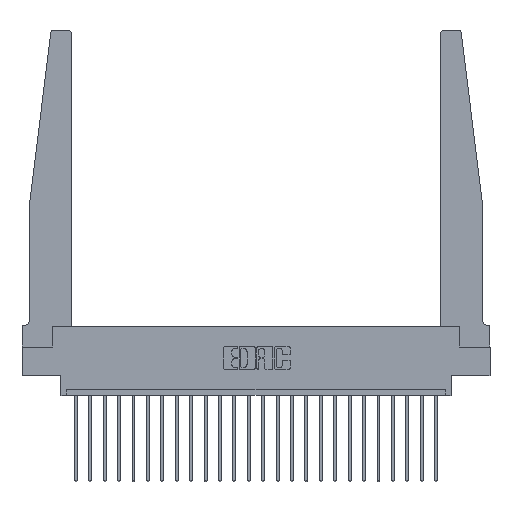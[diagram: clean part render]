
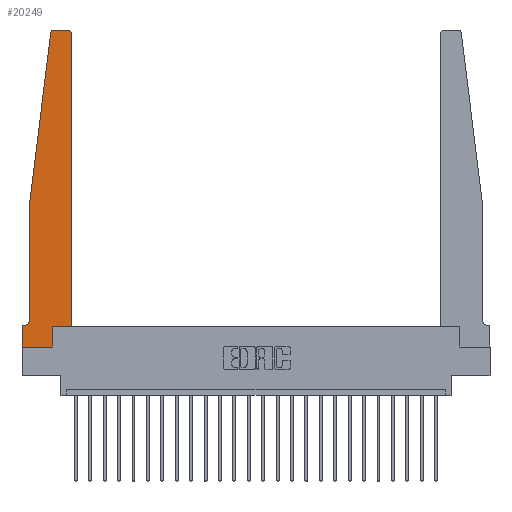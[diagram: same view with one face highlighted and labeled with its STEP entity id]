
A CAD part, top view. The second image highlights one B-rep face of the part: STEP entity #20249.
In plain terms, the highlighted planar face has unit normal (0, 0, 1).
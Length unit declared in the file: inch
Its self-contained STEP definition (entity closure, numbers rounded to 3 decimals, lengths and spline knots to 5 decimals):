
#148 = CARTESIAN_POINT ( 'NONE',  ( 0.24675, 2.72367, 0.37 ) ) ;
#236 = LINE ( 'NONE', #5262, #6137 ) ;
#326 = VERTEX_POINT ( 'NONE', #9006 ) ;
#773 = LINE ( 'NONE', #8058, #2412 ) ;
#903 = VERTEX_POINT ( 'NONE', #23193 ) ;
#1017 = ORIENTED_EDGE ( 'NONE', *, *, #5343, .T. ) ;
#1084 = VERTEX_POINT ( 'NONE', #5472 ) ;
#1524 = EDGE_CURVE ( 'NONE', #8027, #1084, #5301, .T. ) ;
#1527 = EDGE_CURVE ( 'NONE', #903, #20005, #21929, .T. ) ;
#1759 = VERTEX_POINT ( 'NONE', #4455 ) ;
#1843 = CARTESIAN_POINT ( 'NONE',  ( 0.2605, 0., 0.37 ) ) ;
#1944 = CARTESIAN_POINT ( 'NONE',  ( 0., 0., 0.37 ) ) ;
#2383 = DIRECTION ( 'NONE',  ( 0., 1., 0. ) ) ;
#2412 = VECTOR ( 'NONE', #18839, 39.37008 ) ;
#2523 = VECTOR ( 'NONE', #2383, 39.37008 ) ;
#2601 = CARTESIAN_POINT ( 'NONE',  ( 0.065, 0.1875, 0.37 ) ) ;
#2729 = DIRECTION ( 'NONE',  ( 0., 0., 1. ) ) ;
#2732 = DIRECTION ( 'NONE',  ( 0., 0., 1. ) ) ;
#2980 = CARTESIAN_POINT ( 'NONE',  ( 0.27653, 2.72, 0.37 ) ) ;
#3102 = EDGE_CURVE ( 'NONE', #5681, #13576, #7999, .T. ) ;
#3300 = CARTESIAN_POINT ( 'NONE',  ( 0., 0.1875, 0.37 ) ) ;
#3332 = VECTOR ( 'NONE', #19540, 39.37008 ) ;
#3386 = ORIENTED_EDGE ( 'NONE', *, *, #1524, .T. ) ;
#3701 = VECTOR ( 'NONE', #3868, 39.37008 ) ;
#3868 = DIRECTION ( 'NONE',  ( 0., -1., 0. ) ) ;
#3895 = EDGE_CURVE ( 'NONE', #1759, #903, #12063, .T. ) ;
#4279 = EDGE_CURVE ( 'NONE', #1084, #1759, #20562, .T. ) ;
#4455 = CARTESIAN_POINT ( 'NONE',  ( 0.015, 0.1875, 0.37 ) ) ;
#4622 = VERTEX_POINT ( 'NONE', #4796 ) ;
#4790 = CIRCLE ( 'NONE', #18169, 0.03 ) ;
#4796 = CARTESIAN_POINT ( 'NONE',  ( 0.395, 2.75, 0.37 ) ) ;
#4825 = DIRECTION ( 'NONE',  ( -1., 0., 0. ) ) ;
#4871 = FACE_OUTER_BOUND ( 'NONE', #10097, .T. ) ;
#5262 = CARTESIAN_POINT ( 'NONE',  ( 0.425, 0.18, 0.37 ) ) ;
#5301 = LINE ( 'NONE', #5767, #3701 ) ;
#5343 = EDGE_CURVE ( 'NONE', #20005, #5681, #11572, .T. ) ;
#5472 = CARTESIAN_POINT ( 'NONE',  ( 0.065, 0.2375, 0.37 ) ) ;
#5681 = VERTEX_POINT ( 'NONE', #1843 ) ;
#5767 = CARTESIAN_POINT ( 'NONE',  ( 0.065, 1.25, 0.37 ) ) ;
#6028 = LINE ( 'NONE', #11548, #22007 ) ;
#6137 = VECTOR ( 'NONE', #16498, 39.37008 ) ;
#6341 = VECTOR ( 'NONE', #23479, 39.37008 ) ;
#6437 = EDGE_CURVE ( 'NONE', #326, #4622, #4790, .T. ) ;
#7247 = EDGE_CURVE ( 'NONE', #19498, #8027, #6028, .T. ) ;
#7261 = AXIS2_PLACEMENT_3D ( 'NONE', #2980, #2732, #10279 ) ;
#7490 = ORIENTED_EDGE ( 'NONE', *, *, #1527, .T. ) ;
#7635 = CIRCLE ( 'NONE', #7261, 0.03 ) ;
#7999 = LINE ( 'NONE', #11383, #2523 ) ;
#8027 = VERTEX_POINT ( 'NONE', #22631 ) ;
#8058 = CARTESIAN_POINT ( 'NONE',  ( 0.25, 2.75, 0.37 ) ) ;
#8217 = DIRECTION ( 'NONE',  ( -1., 0., 0. ) ) ;
#9006 = CARTESIAN_POINT ( 'NONE',  ( 0.425, 2.72, 0.37 ) ) ;
#9083 = ORIENTED_EDGE ( 'NONE', *, *, #3102, .T. ) ;
#9211 = ORIENTED_EDGE ( 'NONE', *, *, #21481, .T. ) ;
#9898 = CARTESIAN_POINT ( 'NONE',  ( 0.425, 0.18, 0.37 ) ) ;
#10097 = EDGE_LOOP ( 'NONE', ( #18617, #9211, #16314, #3386, #12042, #16622, #7490, #1017, #9083, #17305, #13920, #22218 ) ) ;
#10279 = DIRECTION ( 'NONE',  ( 1., 0., 0. ) ) ;
#11383 = CARTESIAN_POINT ( 'NONE',  ( 0.2605, 0.18, 0.37 ) ) ;
#11409 = EDGE_CURVE ( 'NONE', #4622, #19148, #773, .T. ) ;
#11443 = AXIS2_PLACEMENT_3D ( 'NONE', #3300, #17546, #21727 ) ;
#11548 = CARTESIAN_POINT ( 'NONE',  ( 0.065, 1.25, 0.37 ) ) ;
#11572 = LINE ( 'NONE', #22678, #14547 ) ;
#12042 = ORIENTED_EDGE ( 'NONE', *, *, #4279, .T. ) ;
#12063 = LINE ( 'NONE', #2601, #19394 ) ;
#12240 = DIRECTION ( 'NONE',  ( 0., 0., -1. ) ) ;
#12656 = DIRECTION ( 'NONE',  ( 1., 0., 0. ) ) ;
#13576 = VERTEX_POINT ( 'NONE', #20661 ) ;
#13697 = DIRECTION ( 'NONE',  ( -0.122, -0.992, 0. ) ) ;
#13920 = ORIENTED_EDGE ( 'NONE', *, *, #23523, .T. ) ;
#14271 = CARTESIAN_POINT ( 'NONE',  ( 0.425, 0.18, 0.37 ) ) ;
#14547 = VECTOR ( 'NONE', #19206, 39.37008 ) ;
#15595 = VERTEX_POINT ( 'NONE', #9898 ) ;
#16314 = ORIENTED_EDGE ( 'NONE', *, *, #7247, .T. ) ;
#16498 = DIRECTION ( 'NONE',  ( 0., 1., 0. ) ) ;
#16622 = ORIENTED_EDGE ( 'NONE', *, *, #3895, .T. ) ;
#17305 = ORIENTED_EDGE ( 'NONE', *, *, #17995, .T. ) ;
#17431 = CARTESIAN_POINT ( 'NONE',  ( 0., 0., 0.37 ) ) ;
#17546 = DIRECTION ( 'NONE',  ( 0., 0., 1. ) ) ;
#17861 = LINE ( 'NONE', #14271, #3332 ) ;
#17995 = EDGE_CURVE ( 'NONE', #13576, #15595, #17861, .T. ) ;
#18021 = PLANE ( 'NONE',  #11443 ) ;
#18169 = AXIS2_PLACEMENT_3D ( 'NONE', #19118, #2729, #12656 ) ;
#18617 = ORIENTED_EDGE ( 'NONE', *, *, #11409, .T. ) ;
#18839 = DIRECTION ( 'NONE',  ( -1., 0., 0. ) ) ;
#19118 = CARTESIAN_POINT ( 'NONE',  ( 0.395, 2.72, 0.37 ) ) ;
#19148 = VERTEX_POINT ( 'NONE', #20869 ) ;
#19206 = DIRECTION ( 'NONE',  ( 1., 0., 0. ) ) ;
#19394 = VECTOR ( 'NONE', #8217, 39.37008 ) ;
#19498 = VERTEX_POINT ( 'NONE', #148 ) ;
#19540 = DIRECTION ( 'NONE',  ( 1., 0., 0. ) ) ;
#20005 = VERTEX_POINT ( 'NONE', #17431 ) ;
#20249 = ADVANCED_FACE ( 'NONE', ( #4871 ), #18021, .T. ) ;
#20562 = CIRCLE ( 'NONE', #23594, 0.05 ) ;
#20661 = CARTESIAN_POINT ( 'NONE',  ( 0.2605, 0.18, 0.37 ) ) ;
#20869 = CARTESIAN_POINT ( 'NONE',  ( 0.27653, 2.75, 0.37 ) ) ;
#21332 = CARTESIAN_POINT ( 'NONE',  ( 0.015, 0.2375, 0.37 ) ) ;
#21481 = EDGE_CURVE ( 'NONE', #19148, #19498, #7635, .T. ) ;
#21727 = DIRECTION ( 'NONE',  ( 1., 0., 0. ) ) ;
#21929 = LINE ( 'NONE', #1944, #6341 ) ;
#22007 = VECTOR ( 'NONE', #13697, 39.37008 ) ;
#22218 = ORIENTED_EDGE ( 'NONE', *, *, #6437, .T. ) ;
#22631 = CARTESIAN_POINT ( 'NONE',  ( 0.065, 1.25, 0.37 ) ) ;
#22678 = CARTESIAN_POINT ( 'NONE',  ( 0., 0., 0.37 ) ) ;
#23193 = CARTESIAN_POINT ( 'NONE',  ( 0., 0.1875, 0.37 ) ) ;
#23479 = DIRECTION ( 'NONE',  ( 0., -1., 0. ) ) ;
#23523 = EDGE_CURVE ( 'NONE', #15595, #326, #236, .T. ) ;
#23594 = AXIS2_PLACEMENT_3D ( 'NONE', #21332, #12240, #4825 ) ;
